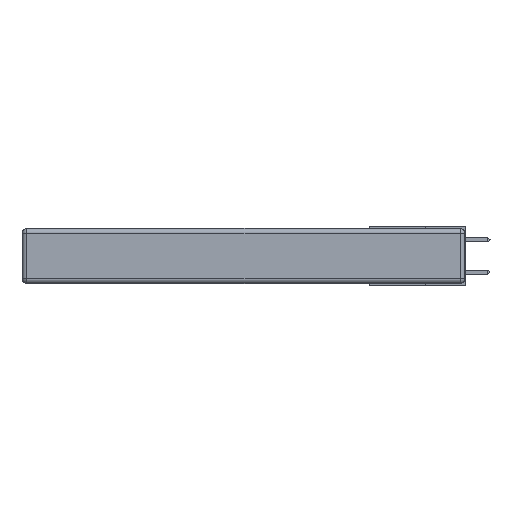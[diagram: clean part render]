
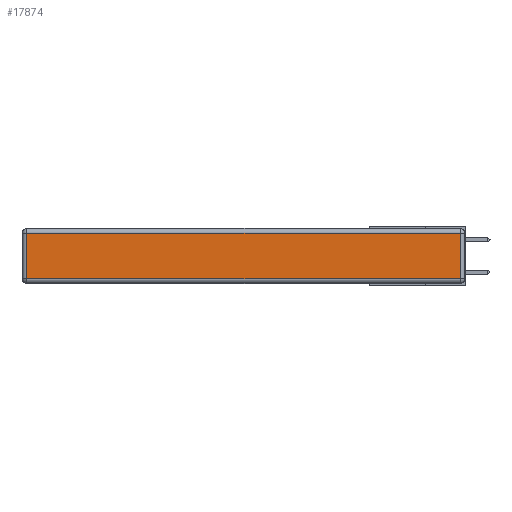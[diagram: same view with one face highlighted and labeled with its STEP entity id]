
A CAD part, left-side view. The second image highlights one B-rep face of the part: STEP entity #17874.
In plain terms, the highlighted planar face has unit normal (-1, 0, 0).
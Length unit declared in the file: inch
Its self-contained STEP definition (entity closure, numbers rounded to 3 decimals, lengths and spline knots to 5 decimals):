
#823 = EDGE_CURVE ( 'NONE', #17083, #13492, #21892, .T. ) ;
#1480 = CARTESIAN_POINT ( 'NONE',  ( 0., 0.03, -0.313 ) ) ;
#1665 = FACE_OUTER_BOUND ( 'NONE', #7472, .T. ) ;
#2740 = VECTOR ( 'NONE', #9005, 39.37008 ) ;
#3204 = VERTEX_POINT ( 'NONE', #17773 ) ;
#4301 = CARTESIAN_POINT ( 'NONE',  ( 0., 2.72, -0.343 ) ) ;
#5230 = VECTOR ( 'NONE', #17230, 39.37008 ) ;
#5258 = LINE ( 'NONE', #9835, #23543 ) ;
#6419 = ORIENTED_EDGE ( 'NONE', *, *, #10725, .T. ) ;
#7472 = EDGE_LOOP ( 'NONE', ( #23845, #23824, #6419, #7814 ) ) ;
#7814 = ORIENTED_EDGE ( 'NONE', *, *, #823, .T. ) ;
#9005 = DIRECTION ( 'NONE',  ( 0., 0., 1. ) ) ;
#9835 = CARTESIAN_POINT ( 'NONE',  ( 0., 2.75, -0.03 ) ) ;
#9986 = DIRECTION ( 'NONE',  ( 0., 1., 0. ) ) ;
#10212 = LINE ( 'NONE', #15341, #5230 ) ;
#10725 = EDGE_CURVE ( 'NONE', #3204, #17083, #5258, .T. ) ;
#11088 = VERTEX_POINT ( 'NONE', #1480 ) ;
#11093 = AXIS2_PLACEMENT_3D ( 'NONE', #23397, #19771, #21461 ) ;
#11134 = EDGE_CURVE ( 'NONE', #13492, #11088, #10212, .T. ) ;
#11579 = VECTOR ( 'NONE', #23125, 39.37008 ) ;
#13492 = VERTEX_POINT ( 'NONE', #14139 ) ;
#14115 = PLANE ( 'NONE',  #11093 ) ;
#14139 = CARTESIAN_POINT ( 'NONE',  ( 0., 2.72, -0.313 ) ) ;
#14365 = EDGE_CURVE ( 'NONE', #11088, #3204, #17721, .T. ) ;
#15341 = CARTESIAN_POINT ( 'NONE',  ( 0., 0., -0.313 ) ) ;
#17083 = VERTEX_POINT ( 'NONE', #17935 ) ;
#17230 = DIRECTION ( 'NONE',  ( 0., -1., 0. ) ) ;
#17721 = LINE ( 'NONE', #24028, #2740 ) ;
#17773 = CARTESIAN_POINT ( 'NONE',  ( 0., 0.03, -0.03 ) ) ;
#17874 = ADVANCED_FACE ( 'NONE', ( #1665 ), #14115, .T. ) ;
#17935 = CARTESIAN_POINT ( 'NONE',  ( 0., 2.72, -0.03 ) ) ;
#19771 = DIRECTION ( 'NONE',  ( -1., 0., 0. ) ) ;
#21461 = DIRECTION ( 'NONE',  ( 0., 0., 1. ) ) ;
#21892 = LINE ( 'NONE', #4301, #11579 ) ;
#23125 = DIRECTION ( 'NONE',  ( 0., 0., -1. ) ) ;
#23397 = CARTESIAN_POINT ( 'NONE',  ( 0., 0., -0.343 ) ) ;
#23543 = VECTOR ( 'NONE', #9986, 39.37008 ) ;
#23824 = ORIENTED_EDGE ( 'NONE', *, *, #14365, .T. ) ;
#23845 = ORIENTED_EDGE ( 'NONE', *, *, #11134, .T. ) ;
#24028 = CARTESIAN_POINT ( 'NONE',  ( 0., 0.03, -0.343 ) ) ;
